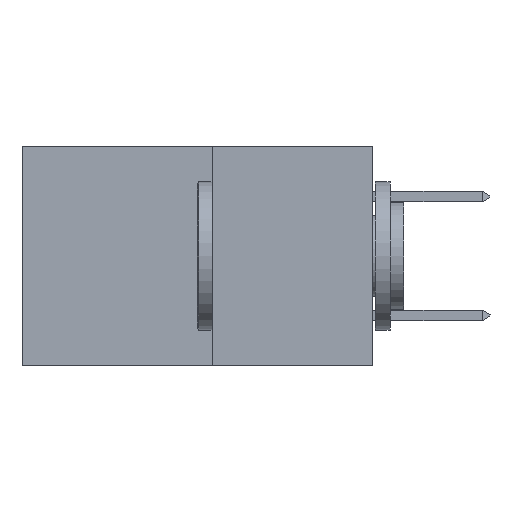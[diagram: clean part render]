
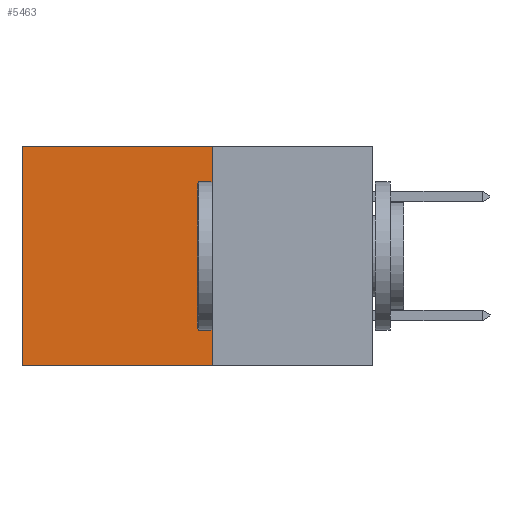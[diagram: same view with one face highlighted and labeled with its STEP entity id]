
A CAD part, left-side view. The second image highlights one B-rep face of the part: STEP entity #5463.
In plain terms, the highlighted planar face has unit normal (-1, 0, 0).
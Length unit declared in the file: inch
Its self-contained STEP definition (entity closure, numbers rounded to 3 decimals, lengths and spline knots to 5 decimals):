
#546 = CARTESIAN_POINT ( 'NONE',  ( 0.277, 0.59, -0.37 ) ) ;
#823 = VERTEX_POINT ( 'NONE', #3485 ) ;
#1303 = EDGE_CURVE ( 'NONE', #30156, #29162, #26408, .T. ) ;
#2609 = DIRECTION ( 'NONE',  ( 0., 1., 0. ) ) ;
#3421 = LINE ( 'NONE', #12950, #29180 ) ;
#3485 = CARTESIAN_POINT ( 'NONE',  ( 0.277, 0.27, -0.37 ) ) ;
#5042 = EDGE_LOOP ( 'NONE', ( #31663, #28557, #28291, #12465 ) ) ;
#5463 = ADVANCED_FACE ( 'NONE', ( #26322 ), #17890, .F. ) ;
#7101 = DIRECTION ( 'NONE',  ( 0., 1., 0. ) ) ;
#9679 = EDGE_CURVE ( 'NONE', #823, #29162, #30454, .T. ) ;
#10304 = CARTESIAN_POINT ( 'NONE',  ( 0.277, 0.27, 0. ) ) ;
#12426 = VECTOR ( 'NONE', #17449, 39.37008 ) ;
#12465 = ORIENTED_EDGE ( 'NONE', *, *, #17716, .T. ) ;
#12950 = CARTESIAN_POINT ( 'NONE',  ( 0.277, 0.27, -0.37 ) ) ;
#14311 = VECTOR ( 'NONE', #2609, 39.37008 ) ;
#14732 = CARTESIAN_POINT ( 'NONE',  ( 0.277, 0.59, -0.37 ) ) ;
#14941 = CARTESIAN_POINT ( 'NONE',  ( 0.277, 0.27, 0. ) ) ;
#17449 = DIRECTION ( 'NONE',  ( 0., 0., -1. ) ) ;
#17716 = EDGE_CURVE ( 'NONE', #27231, #30156, #20917, .T. ) ;
#17814 = DIRECTION ( 'NONE',  ( 0., 0., -1. ) ) ;
#17847 = DIRECTION ( 'NONE',  ( 1., 0., 0. ) ) ;
#17890 = PLANE ( 'NONE',  #27381 ) ;
#18055 = CARTESIAN_POINT ( 'NONE',  ( 0.277, 0.27, -0.37 ) ) ;
#20917 = LINE ( 'NONE', #10304, #14311 ) ;
#23928 = VECTOR ( 'NONE', #7101, 39.37008 ) ;
#26322 = FACE_OUTER_BOUND ( 'NONE', #5042, .T. ) ;
#26408 = LINE ( 'NONE', #546, #12426 ) ;
#27231 = VERTEX_POINT ( 'NONE', #14941 ) ;
#27381 = AXIS2_PLACEMENT_3D ( 'NONE', #18055, #17847, #17814 ) ;
#27802 = DIRECTION ( 'NONE',  ( 0., 0., -1. ) ) ;
#28087 = EDGE_CURVE ( 'NONE', #27231, #823, #3421, .T. ) ;
#28291 = ORIENTED_EDGE ( 'NONE', *, *, #28087, .F. ) ;
#28557 = ORIENTED_EDGE ( 'NONE', *, *, #9679, .F. ) ;
#29162 = VERTEX_POINT ( 'NONE', #14732 ) ;
#29180 = VECTOR ( 'NONE', #27802, 39.37008 ) ;
#29402 = CARTESIAN_POINT ( 'NONE',  ( 0.277, 0.27, -0.37 ) ) ;
#29791 = CARTESIAN_POINT ( 'NONE',  ( 0.277, 0.59, 0. ) ) ;
#30156 = VERTEX_POINT ( 'NONE', #29791 ) ;
#30454 = LINE ( 'NONE', #29402, #23928 ) ;
#31663 = ORIENTED_EDGE ( 'NONE', *, *, #1303, .T. ) ;
